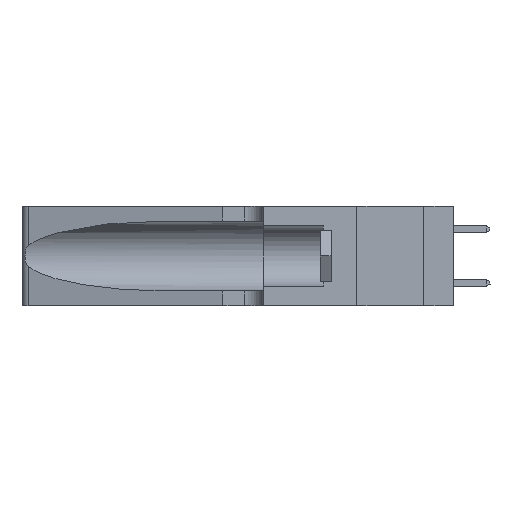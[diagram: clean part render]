
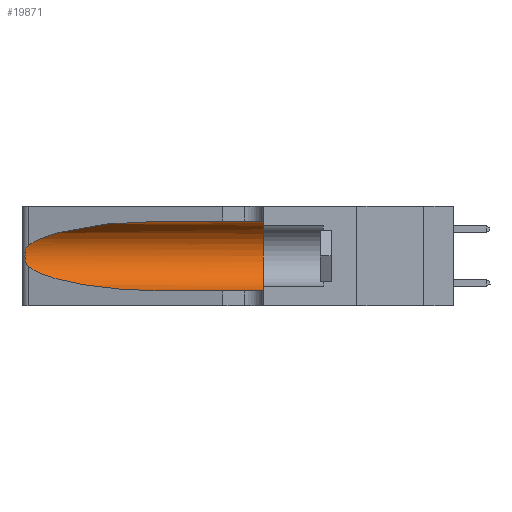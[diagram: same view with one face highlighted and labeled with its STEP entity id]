
A CAD part, left-side view. The second image highlights one B-rep face of the part: STEP entity #19871.
In plain terms, the highlighted cylindrical face has radius 3.308 mm (diameter 6.617 mm), a partial arc.
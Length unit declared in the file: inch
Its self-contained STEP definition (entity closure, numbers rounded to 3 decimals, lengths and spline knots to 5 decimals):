
#586 = CARTESIAN_POINT ( 'NONE',  ( 0.1305, 0.35, 0.05475 ) ) ;
#2547 = CARTESIAN_POINT ( 'NONE',  ( 0.1305, 0.35, 0.185 ) ) ;
#2847 = CARTESIAN_POINT ( 'NONE',  ( 0.2373, 1.15595, 0.28018 ) ) ;
#3207 = CARTESIAN_POINT ( 'NONE',  ( 0.25854, 1.2359, 0.20912 ) ) ;
#4650 = CARTESIAN_POINT ( 'NONE',  ( 0.1305, 0.72297, 0.05475 ) ) ;
#5529 = CARTESIAN_POINT ( 'NONE',  ( 0.1305, 1.61858, 0.31525 ) ) ;
#5624 = VERTEX_POINT ( 'NONE', #586 ) ;
#6369 = DIRECTION ( 'NONE',  ( 0., 0., 1. ) ) ;
#6485 = B_SPLINE_CURVE_WITH_KNOTS ( 'NONE', 3,
 ( #22036, #40907, #10664, #25869, #3207, #29646, #7041, #33446, #10828, #37254, #14621, #41075, #18401, #44824 ),
 .UNSPECIFIED., .F., .F.,
 ( 4, 2, 2, 2, 2, 2, 4 ),
 ( 0., 0.00027, 0.00053, 0.00107, 0.0016, 0.00187, 0.00214 ),
 .UNSPECIFIED. ) ;
#6788 = LINE ( 'NONE', #23453, #25686 ) ;
#7041 = CARTESIAN_POINT ( 'NONE',  ( 0.26075, 1.23896, 0.19203 ) ) ;
#7214 = CARTESIAN_POINT ( 'NONE',  ( 0.1305, 1.61858, 0.185 ) ) ;
#8317 = ORIENTED_EDGE ( 'NONE', *, *, #39166, .F. ) ;
#8859 = ORIENTED_EDGE ( 'NONE', *, *, #47629, .T. ) ;
#9871 = CARTESIAN_POINT ( 'NONE',  ( 0.25487, 1.22718, 0.14631 ) ) ;
#10315 = CARTESIAN_POINT ( 'NONE',  ( 0.1305, 0.72297, 0.31525 ) ) ;
#10664 = CARTESIAN_POINT ( 'NONE',  ( 0.25639, 1.23184, 0.21858 ) ) ;
#10828 = CARTESIAN_POINT ( 'NONE',  ( 0.26017, 1.23833, 0.17102 ) ) ;
#11005 = DIRECTION ( 'NONE',  ( 0., -1., 0. ) ) ;
#11822 = ORIENTED_EDGE ( 'NONE', *, *, #27046, .T. ) ;
#12407 = ORIENTED_EDGE ( 'NONE', *, *, #17154, .T. ) ;
#12475 = CARTESIAN_POINT ( 'NONE',  ( 0.25487, 1.22718, 0.22369 ) ) ;
#14621 = CARTESIAN_POINT ( 'NONE',  ( 0.25789, 1.23486, 0.15765 ) ) ;
#15435 = VERTEX_POINT ( 'NONE', #37464 ) ;
#17154 = EDGE_CURVE ( 'NONE', #38914, #25956, #6485, .T. ) ;
#17292 = CARTESIAN_POINT ( 'NONE',  ( 0.2373, 1.15595, 0.08982 ) ) ;
#17453 = CARTESIAN_POINT ( 'NONE',  ( 0.1305, 0.72297, 0.05475 ) ) ;
#18401 = CARTESIAN_POINT ( 'NONE',  ( 0.25555, 1.22993, 0.14849 ) ) ;
#19871 = ADVANCED_FACE ( 'NONE', ( #47759 ), #46557, .F. ) ;
#22036 = CARTESIAN_POINT ( 'NONE',  ( 0.25487, 1.22718, 0.22369 ) ) ;
#23144 = EDGE_CURVE ( 'NONE', #29748, #5624, #6788, .T. ) ;
#23453 = CARTESIAN_POINT ( 'NONE',  ( 0.1305, 1.61858, 0.05475 ) ) ;
#23482 = EDGE_LOOP ( 'NONE', ( #8859, #12407, #11822, #37883, #8317, #38488 ) ) ;
#25686 = VECTOR ( 'NONE', #38674, 39.37008 ) ;
#25869 = CARTESIAN_POINT ( 'NONE',  ( 0.25787, 1.23484, 0.2124 ) ) ;
#25956 = VERTEX_POINT ( 'NONE', #27873 ) ;
#27046 = EDGE_CURVE ( 'NONE', #25956, #29748, #37969, .T. ) ;
#27357 = LINE ( 'NONE', #5529, #45053 ) ;
#27873 = CARTESIAN_POINT ( 'NONE',  ( 0.25487, 1.22718, 0.14631 ) ) ;
#28957 = DIRECTION ( 'NONE',  ( 0., 1., 0. ) ) ;
#29290 = CARTESIAN_POINT ( 'NONE',  ( 0.25487, 1.22718, 0.22369 ) ) ;
#29646 = CARTESIAN_POINT ( 'NONE',  ( 0.26018, 1.23835, 0.19895 ) ) ;
#29748 = VERTEX_POINT ( 'NONE', #4650 ) ;
#30512 = AXIS2_PLACEMENT_3D ( 'NONE', #2547, #28957, #6369 ) ;
#33446 = CARTESIAN_POINT ( 'NONE',  ( 0.26075, 1.23896, 0.178 ) ) ;
#34376 = CIRCLE ( 'NONE', #30512, 0.13025 ) ;
#35745 = DIRECTION ( 'NONE',  ( 0., -1., 0. ) ) ;
#37254 = CARTESIAN_POINT ( 'NONE',  ( 0.25856, 1.23593, 0.16098 ) ) ;
#37451 = DIRECTION ( 'NONE',  ( 0., 0., -1. ) ) ;
#37464 = CARTESIAN_POINT ( 'NONE',  ( 0.1305, 0.35, 0.31525 ) ) ;
#37883 = ORIENTED_EDGE ( 'NONE', *, *, #23144, .T. ) ;
#37969 =( BOUNDED_CURVE ( )  B_SPLINE_CURVE ( 3, ( #9871, #17292, #40088, #17453 ),
 .UNSPECIFIED., .F., .F. ) 
 B_SPLINE_CURVE_WITH_KNOTS ( ( 4, 4 ),
 ( 3.44316, 4.71239 ),
 .UNSPECIFIED. ) 
 CURVE ( )  GEOMETRIC_REPRESENTATION_ITEM ( )  RATIONAL_B_SPLINE_CURVE ( ( 1., 0.87, 0.87, 1. ) ) 
 REPRESENTATION_ITEM ( '' )  );
#38488 = ORIENTED_EDGE ( 'NONE', *, *, #44335, .F. ) ;
#38674 = DIRECTION ( 'NONE',  ( 0., -1., 0. ) ) ;
#38914 = VERTEX_POINT ( 'NONE', #12475 ) ;
#39166 = EDGE_CURVE ( 'NONE', #15435, #5624, #34376, .T. ) ;
#39505 = AXIS2_PLACEMENT_3D ( 'NONE', #7214, #11005, #37451 ) ;
#40088 = CARTESIAN_POINT ( 'NONE',  ( 0.18966, 0.96281, 0.05475 ) ) ;
#40907 = CARTESIAN_POINT ( 'NONE',  ( 0.25555, 1.22994, 0.2215 ) ) ;
#41075 = CARTESIAN_POINT ( 'NONE',  ( 0.25639, 1.23186, 0.15144 ) ) ;
#43096 =( BOUNDED_CURVE ( )  B_SPLINE_CURVE ( 3, ( #10315, #44297, #2847, #29290 ),
 .UNSPECIFIED., .F., .F. ) 
 B_SPLINE_CURVE_WITH_KNOTS ( ( 4, 4 ),
 ( 1.5708, 2.84003 ),
 .UNSPECIFIED. ) 
 CURVE ( )  GEOMETRIC_REPRESENTATION_ITEM ( )  RATIONAL_B_SPLINE_CURVE ( ( 1., 0.87, 0.87, 1. ) ) 
 REPRESENTATION_ITEM ( '' )  );
#44297 = CARTESIAN_POINT ( 'NONE',  ( 0.18966, 0.96281, 0.31525 ) ) ;
#44335 = EDGE_CURVE ( 'NONE', #48116, #15435, #27357, .T. ) ;
#44824 = CARTESIAN_POINT ( 'NONE',  ( 0.25487, 1.22718, 0.14631 ) ) ;
#45053 = VECTOR ( 'NONE', #35745, 39.37008 ) ;
#46557 = CYLINDRICAL_SURFACE ( 'NONE', #39505, 0.13025 ) ;
#47629 = EDGE_CURVE ( 'NONE', #48116, #38914, #43096, .T. ) ;
#47733 = CARTESIAN_POINT ( 'NONE',  ( 0.1305, 0.72297, 0.31525 ) ) ;
#47759 = FACE_OUTER_BOUND ( 'NONE', #23482, .T. ) ;
#48116 = VERTEX_POINT ( 'NONE', #47733 ) ;
